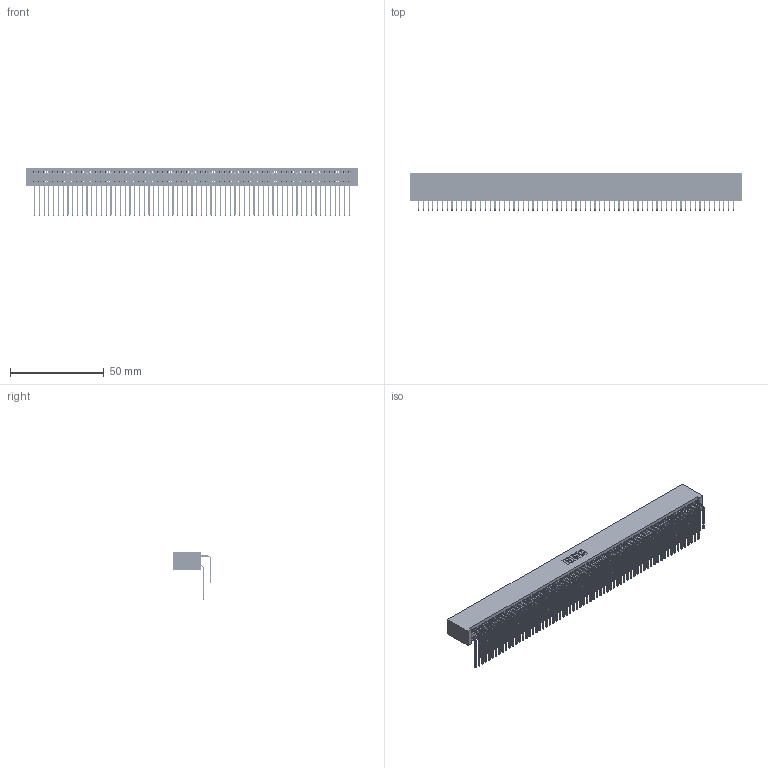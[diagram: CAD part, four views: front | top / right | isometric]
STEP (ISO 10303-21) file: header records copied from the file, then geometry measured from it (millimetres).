
FILE_DESCRIPTION (( 'STEP AP203' ), '1' );
FILE_NAME ('345-134-559-201.STEP', '2018-10-20T11:13:19', ( '' ), ( '' ), 'SwSTEP 2.0', 'SolidWorks 2016', '' );
FILE_SCHEMA (( 'CONFIG_CONTROL_DESIGN' ));
Length unit declared in the file: inch
Products named in the file (4): 345-292-001_558 559 Tail - 1; 345 Part_No Mounting Lugs; 345-292-001_559 Tail - 2; 345-134-559-201
Assembly tree (135 placements, depth 2):
  345-134-559-201
    345 Part_No Mounting Lugs
    345-292-001_558 559 Tail - 1  x67
    345-292-001_559 Tail - 2  x67
Bounding box: 176.78 x 20.56 x 25.53 mm (x, y, z)
Volume: 18794 mm3; surface area: 32203 mm2
Topology: 135 solids, 135 shells, 7086 faces, 21087 edges, 13878 vertices
Faces by surface type: plane 4766, cylinder 2320
Entity records: 50579 total; most frequent: CARTESIAN_POINT 8499, ORIENTED_EDGE 8382, DIRECTION 7431, EDGE_CURVE 4191, LINE 3759, VECTOR 3759, VERTEX_POINT 2790, AXIS2_PLACEMENT_3D 1836
